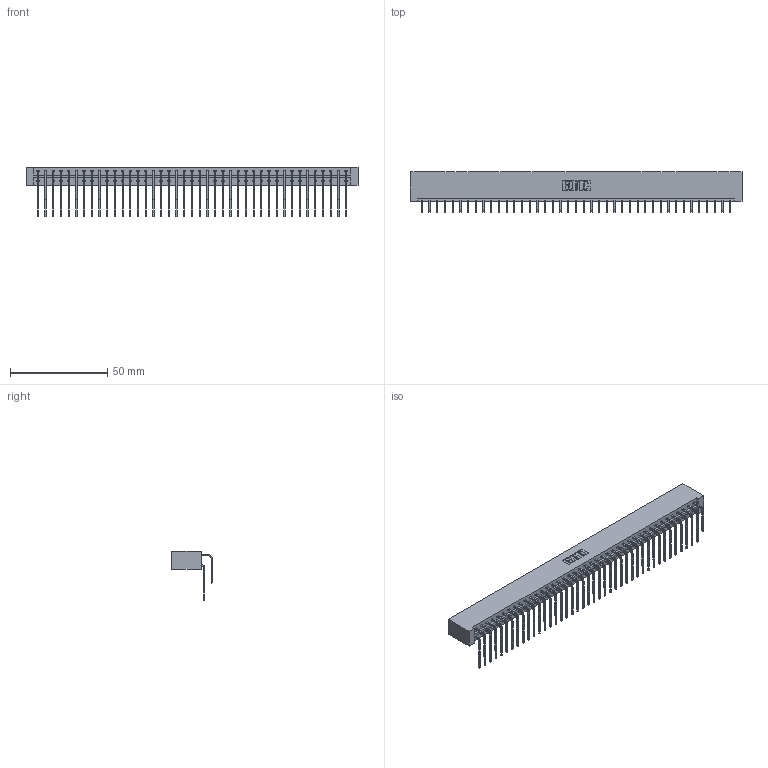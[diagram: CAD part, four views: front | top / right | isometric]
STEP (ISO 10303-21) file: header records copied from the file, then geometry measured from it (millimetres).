
FILE_DESCRIPTION (( 'STEP AP203' ), '1' );
FILE_NAME ('333-082-559-201.STEP', '2018-08-05T03:41:59', ( '' ), ( '' ), 'SwSTEP 2.0', 'SolidWorks 2016', '' );
FILE_SCHEMA (( 'CONFIG_CONTROL_DESIGN' ));
Length unit declared in the file: inch
Products named in the file (4): 333 Part_Lugless; 345-292-001_558 559 Tail - 1; 345-292-001_559 Tail - 2; 333-082-559-201
Assembly tree (83 placements, depth 2):
  333-082-559-201
    333 Part_Lugless
    345-292-001_558 559 Tail - 1  x41
    345-292-001_559 Tail - 2  x41
Bounding box: 170.71 x 20.9 x 25.53 mm (x, y, z)
Volume: 18524.8 mm3; surface area: 24270.7 mm2
Topology: 83 solids, 83 shells, 4534 faces, 13489 edges, 8882 vertices
Faces by surface type: plane 3182, cylinder 1352
Entity records: 28013 total; most frequent: CARTESIAN_POINT 4693, ORIENTED_EDGE 4578, DIRECTION 3985, EDGE_CURVE 2289, LINE 2129, VECTOR 2129, VERTEX_POINT 1522, AXIS2_PLACEMENT_3D 928
